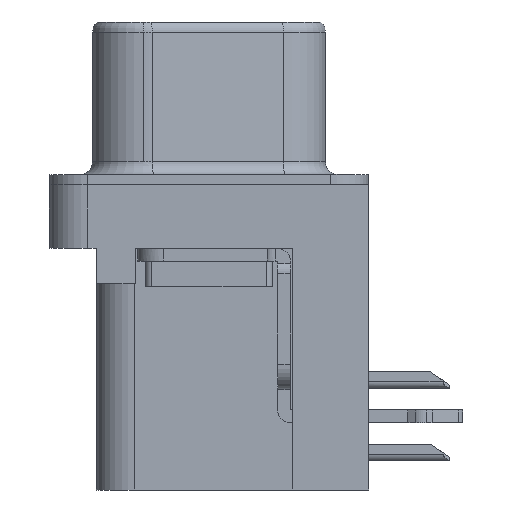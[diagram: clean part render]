
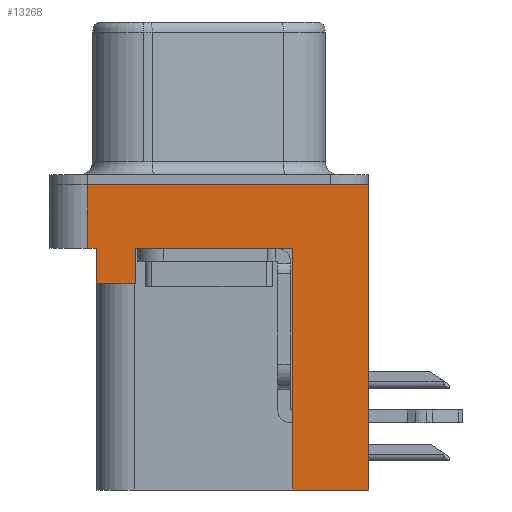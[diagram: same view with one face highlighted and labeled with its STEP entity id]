
A CAD part, left-side view. The second image highlights one B-rep face of the part: STEP entity #13268.
In plain terms, the highlighted planar face has unit normal (-1, 0, 0).
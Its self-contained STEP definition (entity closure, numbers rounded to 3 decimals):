
#25 = ORIENTED_EDGE ( 'NONE', *, *, #3576, .F. ) ;
#350 = DIRECTION ( 'NONE',  ( 0., 0., 1. ) ) ;
#662 = CARTESIAN_POINT ( 'NONE',  ( -2.935, 4.775, -2.5 ) ) ;
#679 = VECTOR ( 'NONE', #9387, 1000. ) ;
#957 = VERTEX_POINT ( 'NONE', #1499 ) ;
#1007 = VERTEX_POINT ( 'NONE', #9862 ) ;
#1036 = EDGE_CURVE ( 'NONE', #1007, #19057, #5723, .T. ) ;
#1101 = LINE ( 'NONE', #4420, #16902 ) ;
#1208 = EDGE_CURVE ( 'NONE', #19057, #17981, #16666, .T. ) ;
#1499 = CARTESIAN_POINT ( 'NONE',  ( -2.935, -6.275, -12. ) ) ;
#1661 = DIRECTION ( 'NONE',  ( 0., 1., 0. ) ) ;
#2203 = LINE ( 'NONE', #4162, #16402 ) ;
#2254 = VECTOR ( 'NONE', #7199, 1000. ) ;
#2382 = CARTESIAN_POINT ( 'NONE',  ( -2.935, 4.425, -3.9 ) ) ;
#2787 = CARTESIAN_POINT ( 'NONE',  ( -2.935, -6.275, -2.5 ) ) ;
#3327 = ORIENTED_EDGE ( 'NONE', *, *, #5137, .T. ) ;
#3576 = EDGE_CURVE ( 'NONE', #17166, #17981, #5925, .T. ) ;
#3603 = ORIENTED_EDGE ( 'NONE', *, *, #17811, .F. ) ;
#3737 = VERTEX_POINT ( 'NONE', #2382 ) ;
#4003 = VECTOR ( 'NONE', #15208, 1000. ) ;
#4147 = CARTESIAN_POINT ( 'NONE',  ( -2.935, -6.275, -2.5 ) ) ;
#4162 = CARTESIAN_POINT ( 'NONE',  ( -2.935, 4.425, -3.9 ) ) ;
#4420 = CARTESIAN_POINT ( 'NONE',  ( -2.935, -6.275, 0. ) ) ;
#4425 = ORIENTED_EDGE ( 'NONE', *, *, #8548, .F. ) ;
#4434 = EDGE_CURVE ( 'NONE', #12196, #16115, #15426, .T. ) ;
#4604 = DIRECTION ( 'NONE',  ( 0., -1., 0. ) ) ;
#4771 = CARTESIAN_POINT ( 'NONE',  ( -2.935, -6.275, -2.5 ) ) ;
#5028 = ORIENTED_EDGE ( 'NONE', *, *, #14268, .F. ) ;
#5137 = EDGE_CURVE ( 'NONE', #12196, #8292, #7948, .T. ) ;
#5438 = VECTOR ( 'NONE', #13742, 1000. ) ;
#5494 = VECTOR ( 'NONE', #350, 1000. ) ;
#5723 = LINE ( 'NONE', #16240, #12015 ) ;
#5866 = CARTESIAN_POINT ( 'NONE',  ( -2.935, -3.295, -12. ) ) ;
#5915 = CARTESIAN_POINT ( 'NONE',  ( -2.935, -3.295, -12. ) ) ;
#5925 = LINE ( 'NONE', #17885, #12418 ) ;
#6241 = FACE_OUTER_BOUND ( 'NONE', #17575, .T. ) ;
#7103 = CARTESIAN_POINT ( 'NONE',  ( -2.935, 2.895, -2.5 ) ) ;
#7199 = DIRECTION ( 'NONE',  ( 0., -1., 0. ) ) ;
#7894 = LINE ( 'NONE', #5915, #19302 ) ;
#7909 = LINE ( 'NONE', #4771, #679 ) ;
#7948 = LINE ( 'NONE', #2787, #4003 ) ;
#8105 = ORIENTED_EDGE ( 'NONE', *, *, #1208, .T. ) ;
#8292 = VERTEX_POINT ( 'NONE', #10843 ) ;
#8336 = CARTESIAN_POINT ( 'NONE',  ( -2.935, -6.275, 0. ) ) ;
#8548 = EDGE_CURVE ( 'NONE', #16115, #16362, #1101, .T. ) ;
#9387 = DIRECTION ( 'NONE',  ( 0., 0., 1. ) ) ;
#9862 = CARTESIAN_POINT ( 'NONE',  ( -2.935, 2.895, -3.9 ) ) ;
#10265 = DIRECTION ( 'NONE',  ( 0., 1., 0. ) ) ;
#10679 = CARTESIAN_POINT ( 'NONE',  ( -2.935, -6.275, -2.5 ) ) ;
#10830 = ORIENTED_EDGE ( 'NONE', *, *, #4434, .F. ) ;
#10843 = CARTESIAN_POINT ( 'NONE',  ( -2.935, 4.425, -2.5 ) ) ;
#11833 = DIRECTION ( 'NONE',  ( 0., 0., 1. ) ) ;
#12015 = VECTOR ( 'NONE', #11833, 1000. ) ;
#12129 = EDGE_CURVE ( 'NONE', #957, #16362, #7909, .T. ) ;
#12196 = VERTEX_POINT ( 'NONE', #19176 ) ;
#12417 = EDGE_CURVE ( 'NONE', #957, #17166, #7894, .T. ) ;
#12418 = VECTOR ( 'NONE', #17949, 1000. ) ;
#12715 = ORIENTED_EDGE ( 'NONE', *, *, #12417, .F. ) ;
#13268 = ADVANCED_FACE ( 'NONE', ( #6241 ), #15357, .T. ) ;
#13494 = ORIENTED_EDGE ( 'NONE', *, *, #12129, .T. ) ;
#13742 = DIRECTION ( 'NONE',  ( 0., 0., 1. ) ) ;
#13769 = CARTESIAN_POINT ( 'NONE',  ( -2.935, 4.425, -3.9 ) ) ;
#14268 = EDGE_CURVE ( 'NONE', #3737, #8292, #19227, .T. ) ;
#14570 = AXIS2_PLACEMENT_3D ( 'NONE', #10679, #16715, #16908 ) ;
#14800 = CARTESIAN_POINT ( 'NONE',  ( -2.935, -3.295, -2.5 ) ) ;
#15208 = DIRECTION ( 'NONE',  ( 0., -1., 0. ) ) ;
#15357 = PLANE ( 'NONE',  #14570 ) ;
#15426 = LINE ( 'NONE', #662, #5438 ) ;
#16115 = VERTEX_POINT ( 'NONE', #18080 ) ;
#16240 = CARTESIAN_POINT ( 'NONE',  ( -2.935, 2.895, -3.9 ) ) ;
#16362 = VERTEX_POINT ( 'NONE', #8336 ) ;
#16402 = VECTOR ( 'NONE', #10265, 1000. ) ;
#16649 = ORIENTED_EDGE ( 'NONE', *, *, #1036, .T. ) ;
#16666 = LINE ( 'NONE', #4147, #2254 ) ;
#16715 = DIRECTION ( 'NONE',  ( -1., 0., 0. ) ) ;
#16902 = VECTOR ( 'NONE', #4604, 1000. ) ;
#16908 = DIRECTION ( 'NONE',  ( 0., 0., 1. ) ) ;
#17166 = VERTEX_POINT ( 'NONE', #5866 ) ;
#17575 = EDGE_LOOP ( 'NONE', ( #4425, #10830, #3327, #5028, #3603, #16649, #8105, #25, #12715, #13494 ) ) ;
#17811 = EDGE_CURVE ( 'NONE', #1007, #3737, #2203, .T. ) ;
#17885 = CARTESIAN_POINT ( 'NONE',  ( -2.935, -3.295, -12. ) ) ;
#17949 = DIRECTION ( 'NONE',  ( 0., 0., 1. ) ) ;
#17981 = VERTEX_POINT ( 'NONE', #14800 ) ;
#18080 = CARTESIAN_POINT ( 'NONE',  ( -2.935, 4.775, 0. ) ) ;
#19057 = VERTEX_POINT ( 'NONE', #7103 ) ;
#19176 = CARTESIAN_POINT ( 'NONE',  ( -2.935, 4.775, -2.5 ) ) ;
#19227 = LINE ( 'NONE', #13769, #5494 ) ;
#19302 = VECTOR ( 'NONE', #1661, 1000. ) ;
